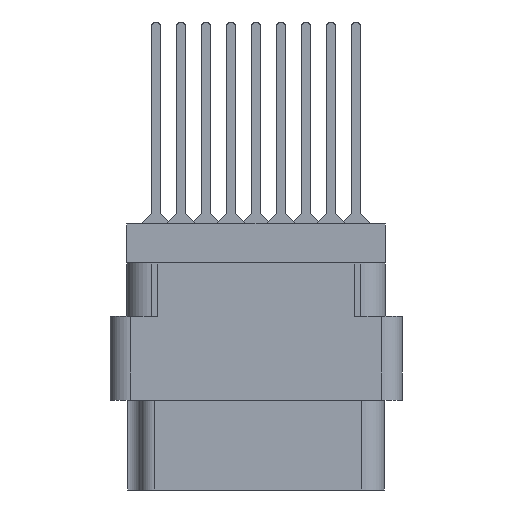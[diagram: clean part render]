
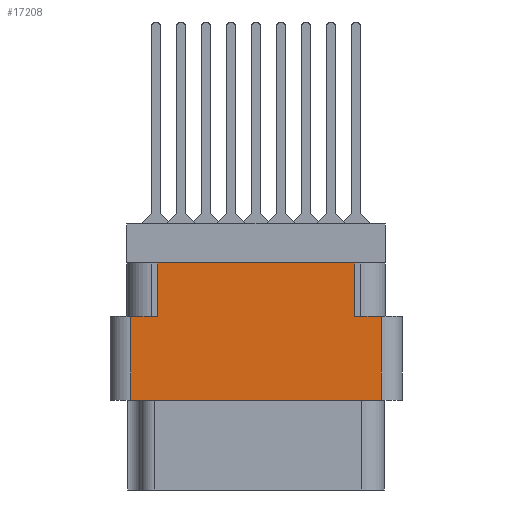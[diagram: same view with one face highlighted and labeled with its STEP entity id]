
A CAD part, left-side view. The second image highlights one B-rep face of the part: STEP entity #17208.
In plain terms, the highlighted planar face has unit normal (-1, 0, 0).
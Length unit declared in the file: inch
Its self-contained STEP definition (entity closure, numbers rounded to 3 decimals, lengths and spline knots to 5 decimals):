
#202 = DIRECTION ( 'NONE',  ( 0., 0., 1. ) ) ;
#611 = LINE ( 'NONE', #677, #15626 ) ;
#677 = CARTESIAN_POINT ( 'NONE',  ( -1., 0.296, -0.277 ) ) ;
#2633 = DIRECTION ( 'NONE',  ( 0., 0., 1. ) ) ;
#4779 = VECTOR ( 'NONE', #5390, 39.37008 ) ;
#5273 = DIRECTION ( 'NONE',  ( 0., 0., 1. ) ) ;
#5390 = DIRECTION ( 'NONE',  ( 0., 1., 0. ) ) ;
#5710 = EDGE_CURVE ( 'NONE', #15892, #21888, #22775, .T. ) ;
#7490 = LINE ( 'NONE', #25981, #28466 ) ;
#7866 = EDGE_CURVE ( 'NONE', #10652, #13452, #34075, .T. ) ;
#7905 = AXIS2_PLACEMENT_3D ( 'NONE', #16180, #29631, #202 ) ;
#8313 = CARTESIAN_POINT ( 'NONE',  ( -1., 0.376, -0.798 ) ) ;
#8978 = ORIENTED_EDGE ( 'NONE', *, *, #32462, .T. ) ;
#10652 = VERTEX_POINT ( 'NONE', #23445 ) ;
#10780 = LINE ( 'NONE', #8313, #31362 ) ;
#10786 = CARTESIAN_POINT ( 'NONE',  ( -1., 0.376, -0.529 ) ) ;
#10839 = PLANE ( 'NONE',  #7905 ) ;
#11341 = DIRECTION ( 'NONE',  ( 0., -1., 0. ) ) ;
#11653 = VECTOR ( 'NONE', #11341, 39.37008 ) ;
#12365 = FACE_OUTER_BOUND ( 'NONE', #30520, .T. ) ;
#12543 = DIRECTION ( 'NONE',  ( 0., -1., 0. ) ) ;
#12978 = CARTESIAN_POINT ( 'NONE',  ( -1., -0.376, -0.277 ) ) ;
#13011 = CARTESIAN_POINT ( 'NONE',  ( -1., -0.376, -0.529 ) ) ;
#13452 = VERTEX_POINT ( 'NONE', #28399 ) ;
#13660 = DIRECTION ( 'NONE',  ( 0., 0., -1. ) ) ;
#13898 = CARTESIAN_POINT ( 'NONE',  ( -1., 0.296, -0.277 ) ) ;
#15466 = ORIENTED_EDGE ( 'NONE', *, *, #31984, .F. ) ;
#15626 = VECTOR ( 'NONE', #27053, 39.37008 ) ;
#15743 = ORIENTED_EDGE ( 'NONE', *, *, #5710, .F. ) ;
#15892 = VERTEX_POINT ( 'NONE', #13011 ) ;
#15949 = EDGE_CURVE ( 'NONE', #32543, #13452, #7490, .T. ) ;
#16180 = CARTESIAN_POINT ( 'NONE',  ( -1., -0.438, -0.798 ) ) ;
#16785 = LINE ( 'NONE', #21012, #18889 ) ;
#16804 = VERTEX_POINT ( 'NONE', #28130 ) ;
#17208 = ADVANCED_FACE ( 'NONE', ( #12365 ), #10839, .T. ) ;
#18257 = EDGE_CURVE ( 'NONE', #29106, #32543, #611, .T. ) ;
#18425 = LINE ( 'NONE', #26729, #24338 ) ;
#18889 = VECTOR ( 'NONE', #28800, 39.37008 ) ;
#21012 = CARTESIAN_POINT ( 'NONE',  ( -1., 0., -0.277 ) ) ;
#21888 = VERTEX_POINT ( 'NONE', #10786 ) ;
#22775 = LINE ( 'NONE', #29197, #4779 ) ;
#23445 = CARTESIAN_POINT ( 'NONE',  ( -1., -0.296, -0.277 ) ) ;
#24338 = VECTOR ( 'NONE', #5273, 39.37008 ) ;
#24490 = ORIENTED_EDGE ( 'NONE', *, *, #15949, .F. ) ;
#25103 = LINE ( 'NONE', #30251, #11653 ) ;
#25981 = CARTESIAN_POINT ( 'NONE',  ( -1., 0.438, -0.117 ) ) ;
#26113 = ORIENTED_EDGE ( 'NONE', *, *, #18257, .F. ) ;
#26729 = CARTESIAN_POINT ( 'NONE',  ( -1., -0.376, -0.798 ) ) ;
#27053 = DIRECTION ( 'NONE',  ( 0., 0., 1. ) ) ;
#28130 = CARTESIAN_POINT ( 'NONE',  ( -1., 0.376, -0.277 ) ) ;
#28399 = CARTESIAN_POINT ( 'NONE',  ( -1., -0.296, -0.117 ) ) ;
#28466 = VECTOR ( 'NONE', #12543, 39.37008 ) ;
#28628 = VECTOR ( 'NONE', #2633, 39.37008 ) ;
#28800 = DIRECTION ( 'NONE',  ( 0., -1., 0. ) ) ;
#29106 = VERTEX_POINT ( 'NONE', #13898 ) ;
#29197 = CARTESIAN_POINT ( 'NONE',  ( -1., 0., -0.529 ) ) ;
#29380 = EDGE_CURVE ( 'NONE', #16804, #29106, #16785, .T. ) ;
#29631 = DIRECTION ( 'NONE',  ( -1., 0., 0. ) ) ;
#30251 = CARTESIAN_POINT ( 'NONE',  ( -1., 0., -0.277 ) ) ;
#30466 = CARTESIAN_POINT ( 'NONE',  ( -1., 0.296, -0.117 ) ) ;
#30520 = EDGE_LOOP ( 'NONE', ( #34739, #8978, #15743, #30844, #15466, #33925, #24490, #26113 ) ) ;
#30844 = ORIENTED_EDGE ( 'NONE', *, *, #34172, .T. ) ;
#31362 = VECTOR ( 'NONE', #13660, 39.37008 ) ;
#31704 = VERTEX_POINT ( 'NONE', #12978 ) ;
#31984 = EDGE_CURVE ( 'NONE', #10652, #31704, #25103, .T. ) ;
#32029 = CARTESIAN_POINT ( 'NONE',  ( -1., -0.296, -0.277 ) ) ;
#32462 = EDGE_CURVE ( 'NONE', #16804, #21888, #10780, .T. ) ;
#32543 = VERTEX_POINT ( 'NONE', #30466 ) ;
#33925 = ORIENTED_EDGE ( 'NONE', *, *, #7866, .T. ) ;
#34075 = LINE ( 'NONE', #32029, #28628 ) ;
#34172 = EDGE_CURVE ( 'NONE', #15892, #31704, #18425, .T. ) ;
#34739 = ORIENTED_EDGE ( 'NONE', *, *, #29380, .F. ) ;
